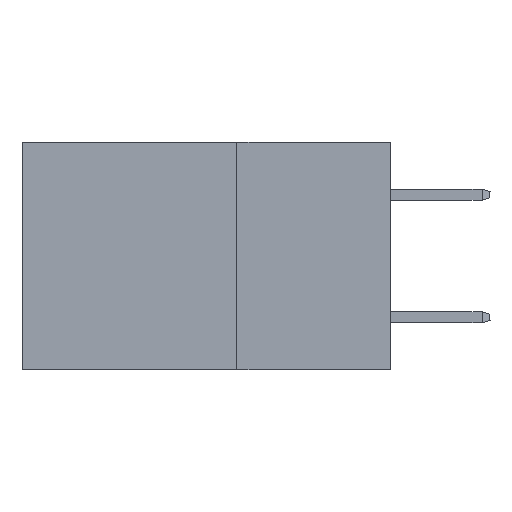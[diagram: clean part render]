
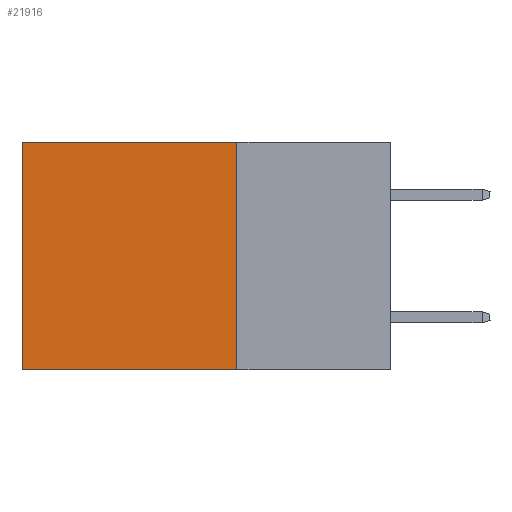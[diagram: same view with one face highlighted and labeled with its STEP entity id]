
A CAD part, left-side view. The second image highlights one B-rep face of the part: STEP entity #21916.
In plain terms, the highlighted planar face has unit normal (-1, 0, 0).
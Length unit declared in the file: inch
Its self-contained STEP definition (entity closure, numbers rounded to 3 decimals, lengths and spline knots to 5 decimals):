
#3 = CARTESIAN_POINT ( 'NONE',  ( 0.2875, 0.25, -0.37 ) ) ;
#721 = VERTEX_POINT ( 'NONE', #7963 ) ;
#1103 = VERTEX_POINT ( 'NONE', #9435 ) ;
#2116 = VECTOR ( 'NONE', #25437, 39.37008 ) ;
#2702 = CARTESIAN_POINT ( 'NONE',  ( 0.2875, 0.6, 0. ) ) ;
#2912 = EDGE_CURVE ( 'NONE', #1103, #721, #10900, .T. ) ;
#3770 = PLANE ( 'NONE',  #33127 ) ;
#5740 = DIRECTION ( 'NONE',  ( 0., 1., 0. ) ) ;
#7963 = CARTESIAN_POINT ( 'NONE',  ( 0.2875, 0.25, -0.37 ) ) ;
#8322 = ORIENTED_EDGE ( 'NONE', *, *, #17704, .T. ) ;
#8444 = LINE ( 'NONE', #3, #13769 ) ;
#8584 = DIRECTION ( 'NONE',  ( 0., 0., -1. ) ) ;
#9007 = EDGE_CURVE ( 'NONE', #721, #35003, #8444, .T. ) ;
#9435 = CARTESIAN_POINT ( 'NONE',  ( 0.2875, 0.25, 0. ) ) ;
#9459 = CARTESIAN_POINT ( 'NONE',  ( 0.2875, 0.6, 0. ) ) ;
#10577 = EDGE_CURVE ( 'NONE', #1103, #18722, #33348, .T. ) ;
#10900 = LINE ( 'NONE', #25831, #22989 ) ;
#11390 = ORIENTED_EDGE ( 'NONE', *, *, #9007, .F. ) ;
#13769 = VECTOR ( 'NONE', #5740, 39.37008 ) ;
#14271 = CARTESIAN_POINT ( 'NONE',  ( 0.2875, 0.25, 0. ) ) ;
#15454 = CARTESIAN_POINT ( 'NONE',  ( 0.2875, 0.25, 0. ) ) ;
#15586 = DIRECTION ( 'NONE',  ( 0., 0., -1. ) ) ;
#17704 = EDGE_CURVE ( 'NONE', #18722, #35003, #25145, .T. ) ;
#18454 = DIRECTION ( 'NONE',  ( 1., 0., 0. ) ) ;
#18722 = VERTEX_POINT ( 'NONE', #2702 ) ;
#21916 = ADVANCED_FACE ( 'NONE', ( #35747 ), #3770, .F. ) ;
#22989 = VECTOR ( 'NONE', #8584, 39.37008 ) ;
#24239 = VECTOR ( 'NONE', #29818, 39.37008 ) ;
#25145 = LINE ( 'NONE', #9459, #24239 ) ;
#25437 = DIRECTION ( 'NONE',  ( 0., 1., 0. ) ) ;
#25831 = CARTESIAN_POINT ( 'NONE',  ( 0.2875, 0.25, 0. ) ) ;
#26799 = ORIENTED_EDGE ( 'NONE', *, *, #10577, .T. ) ;
#29377 = ORIENTED_EDGE ( 'NONE', *, *, #2912, .F. ) ;
#29818 = DIRECTION ( 'NONE',  ( 0., 0., -1. ) ) ;
#31561 = CARTESIAN_POINT ( 'NONE',  ( 0.2875, 0.6, -0.37 ) ) ;
#32462 = EDGE_LOOP ( 'NONE', ( #8322, #11390, #29377, #26799 ) ) ;
#33127 = AXIS2_PLACEMENT_3D ( 'NONE', #15454, #18454, #15586 ) ;
#33348 = LINE ( 'NONE', #14271, #2116 ) ;
#35003 = VERTEX_POINT ( 'NONE', #31561 ) ;
#35747 = FACE_OUTER_BOUND ( 'NONE', #32462, .T. ) ;
